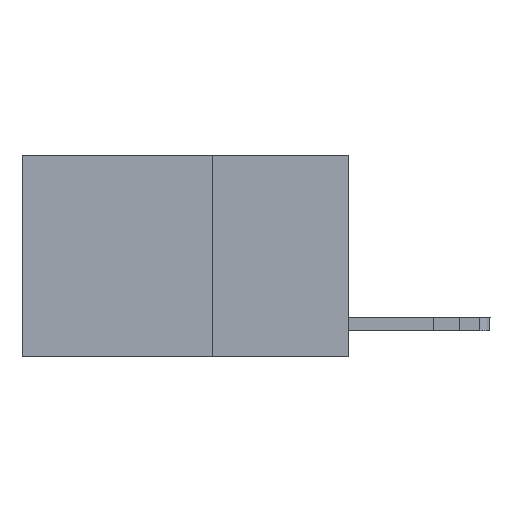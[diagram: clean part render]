
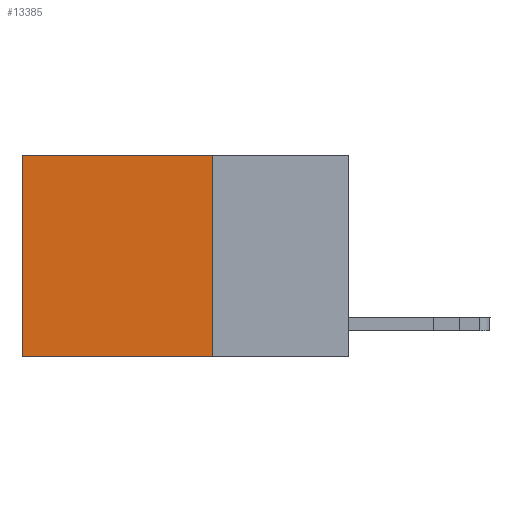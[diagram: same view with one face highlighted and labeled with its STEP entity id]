
A CAD part, left-side view. The second image highlights one B-rep face of the part: STEP entity #13385.
In plain terms, the highlighted planar face has unit normal (-1, 0, 0).
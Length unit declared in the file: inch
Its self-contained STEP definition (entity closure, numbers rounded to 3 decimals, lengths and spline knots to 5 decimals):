
#228 = ORIENTED_EDGE ( 'NONE', *, *, #3078, .F. ) ;
#988 = LINE ( 'NONE', #16280, #14383 ) ;
#1381 = DIRECTION ( 'NONE',  ( 0., 0., -1. ) ) ;
#1658 = ORIENTED_EDGE ( 'NONE', *, *, #8786, .T. ) ;
#2126 = VERTEX_POINT ( 'NONE', #14058 ) ;
#2132 = VERTEX_POINT ( 'NONE', #14042 ) ;
#2499 = CARTESIAN_POINT ( 'NONE',  ( 0.2625, 0.6, 0. ) ) ;
#2594 = CARTESIAN_POINT ( 'NONE',  ( 0.2625, 0.25, -0.37 ) ) ;
#2595 = CARTESIAN_POINT ( 'NONE',  ( 0.2625, 0.25, 0. ) ) ;
#2612 = DIRECTION ( 'NONE',  ( 0., 1., 0. ) ) ;
#3078 = EDGE_CURVE ( 'NONE', #2126, #2132, #4065, .T. ) ;
#3651 = VECTOR ( 'NONE', #2612, 39.37008 ) ;
#3663 = DIRECTION ( 'NONE',  ( 0., 0., -1. ) ) ;
#4065 = LINE ( 'NONE', #2594, #3651 ) ;
#4172 = VECTOR ( 'NONE', #1381, 39.37008 ) ;
#4956 = VERTEX_POINT ( 'NONE', #2595 ) ;
#5755 = CARTESIAN_POINT ( 'NONE',  ( 0.2625, 0.25, 0. ) ) ;
#6248 = VERTEX_POINT ( 'NONE', #2499 ) ;
#6704 = FACE_OUTER_BOUND ( 'NONE', #12807, .T. ) ;
#7030 = DIRECTION ( 'NONE',  ( 0., 0., -1. ) ) ;
#7453 = LINE ( 'NONE', #8722, #10461 ) ;
#7523 = LINE ( 'NONE', #10511, #4172 ) ;
#8138 = ORIENTED_EDGE ( 'NONE', *, *, #14840, .T. ) ;
#8722 = CARTESIAN_POINT ( 'NONE',  ( 0.2625, 0.6, 0. ) ) ;
#8786 = EDGE_CURVE ( 'NONE', #6248, #2132, #7453, .T. ) ;
#10302 = AXIS2_PLACEMENT_3D ( 'NONE', #5755, #14629, #7030 ) ;
#10461 = VECTOR ( 'NONE', #3663, 39.37008 ) ;
#10511 = CARTESIAN_POINT ( 'NONE',  ( 0.2625, 0.25, 0. ) ) ;
#12358 = EDGE_CURVE ( 'NONE', #4956, #2126, #7523, .T. ) ;
#12559 = DIRECTION ( 'NONE',  ( 0., 1., 0. ) ) ;
#12807 = EDGE_LOOP ( 'NONE', ( #1658, #228, #16062, #8138 ) ) ;
#13385 = ADVANCED_FACE ( 'NONE', ( #6704 ), #15843, .F. ) ;
#14042 = CARTESIAN_POINT ( 'NONE',  ( 0.2625, 0.6, -0.37 ) ) ;
#14058 = CARTESIAN_POINT ( 'NONE',  ( 0.2625, 0.25, -0.37 ) ) ;
#14383 = VECTOR ( 'NONE', #12559, 39.37008 ) ;
#14629 = DIRECTION ( 'NONE',  ( 1., 0., 0. ) ) ;
#14840 = EDGE_CURVE ( 'NONE', #4956, #6248, #988, .T. ) ;
#15843 = PLANE ( 'NONE',  #10302 ) ;
#16062 = ORIENTED_EDGE ( 'NONE', *, *, #12358, .F. ) ;
#16280 = CARTESIAN_POINT ( 'NONE',  ( 0.2625, 0.25, 0. ) ) ;
